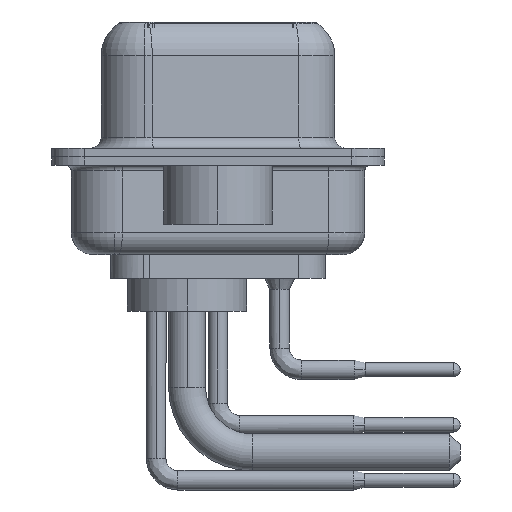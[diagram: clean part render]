
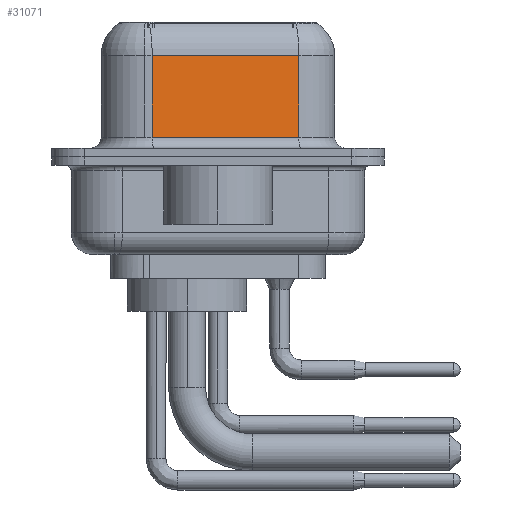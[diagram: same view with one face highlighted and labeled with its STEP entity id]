
A CAD part, left-side view. The second image highlights one B-rep face of the part: STEP entity #31071.
In plain terms, the highlighted planar face has unit normal (-0.985, -0.174, 0).
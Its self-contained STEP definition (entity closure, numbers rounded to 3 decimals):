
#340 = DIRECTION ( 'NONE',  ( -0.174, 0.985, 0. ) ) ;
#516 = CARTESIAN_POINT ( 'NONE',  ( 5.621, -3.722, 4.65 ) ) ;
#856 = LINE ( 'NONE', #516, #23020 ) ;
#1718 = EDGE_CURVE ( 'NONE', #20578, #8734, #25523, .T. ) ;
#2803 = LINE ( 'NONE', #16384, #6237 ) ;
#5321 = ORIENTED_EDGE ( 'NONE', *, *, #1718, .F. ) ;
#5566 = CARTESIAN_POINT ( 'NONE',  ( 5.621, -3.722, 4.65 ) ) ;
#5639 = VERTEX_POINT ( 'NONE', #33700 ) ;
#6237 = VECTOR ( 'NONE', #23940, 1000. ) ;
#6823 = CARTESIAN_POINT ( 'NONE',  ( 5.621, -3.722, 0.9 ) ) ;
#8734 = VERTEX_POINT ( 'NONE', #24320 ) ;
#10242 = EDGE_CURVE ( 'NONE', #30274, #5639, #2803, .T. ) ;
#10982 = EDGE_LOOP ( 'NONE', ( #5321, #31204, #16221, #11341 ) ) ;
#11341 = ORIENTED_EDGE ( 'NONE', *, *, #23833, .T. ) ;
#11877 = FACE_OUTER_BOUND ( 'NONE', #10982, .T. ) ;
#12642 = AXIS2_PLACEMENT_3D ( 'NONE', #20148, #22880, #19803 ) ;
#14870 = DIRECTION ( 'NONE',  ( 0., 0., -1. ) ) ;
#16221 = ORIENTED_EDGE ( 'NONE', *, *, #10242, .T. ) ;
#16384 = CARTESIAN_POINT ( 'NONE',  ( 4.43, 3.028, 6.4 ) ) ;
#17636 = VECTOR ( 'NONE', #19553, 1000. ) ;
#17970 = CARTESIAN_POINT ( 'NONE',  ( 5.621, -3.722, 6.4 ) ) ;
#19553 = DIRECTION ( 'NONE',  ( 0.174, -0.985, 0. ) ) ;
#19803 = DIRECTION ( 'NONE',  ( -0.174, 0.985, 0. ) ) ;
#20148 = CARTESIAN_POINT ( 'NONE',  ( 5.621, -3.722, 6.4 ) ) ;
#20578 = VERTEX_POINT ( 'NONE', #5566 ) ;
#22371 = PLANE ( 'NONE',  #12642 ) ;
#22880 = DIRECTION ( 'NONE',  ( 0.985, 0.174, 0. ) ) ;
#23020 = VECTOR ( 'NONE', #340, 1000. ) ;
#23833 = EDGE_CURVE ( 'NONE', #5639, #8734, #27930, .T. ) ;
#23940 = DIRECTION ( 'NONE',  ( 0., 0., -1. ) ) ;
#24320 = CARTESIAN_POINT ( 'NONE',  ( 5.621, -3.722, 0.9 ) ) ;
#25523 = LINE ( 'NONE', #17970, #25862 ) ;
#25862 = VECTOR ( 'NONE', #14870, 1000. ) ;
#27930 = LINE ( 'NONE', #6823, #17636 ) ;
#30111 = EDGE_CURVE ( 'NONE', #20578, #30274, #856, .T. ) ;
#30196 = CARTESIAN_POINT ( 'NONE',  ( 4.43, 3.028, 4.65 ) ) ;
#30274 = VERTEX_POINT ( 'NONE', #30196 ) ;
#31071 = ADVANCED_FACE ( 'NONE', ( #11877 ), #22371, .F. ) ;
#31204 = ORIENTED_EDGE ( 'NONE', *, *, #30111, .T. ) ;
#33700 = CARTESIAN_POINT ( 'NONE',  ( 4.43, 3.028, 0.9 ) ) ;
